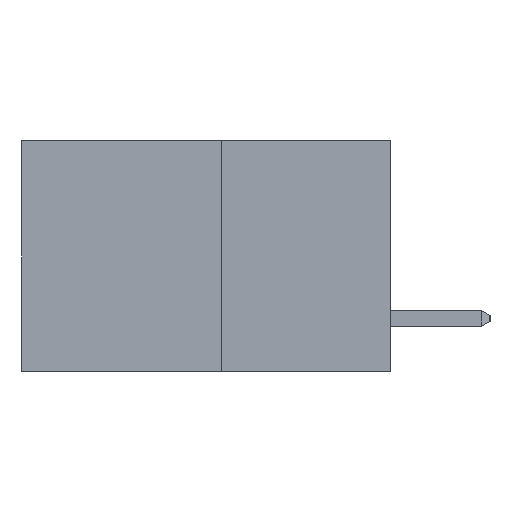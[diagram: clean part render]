
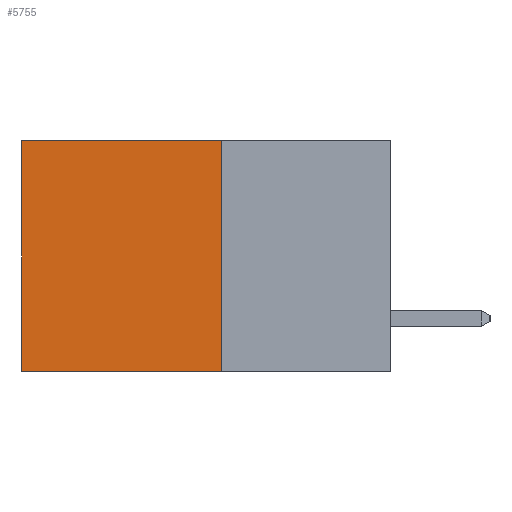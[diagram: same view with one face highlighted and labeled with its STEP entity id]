
A CAD part, left-side view. The second image highlights one B-rep face of the part: STEP entity #5755.
In plain terms, the highlighted planar face has unit normal (-1, 0, 0).
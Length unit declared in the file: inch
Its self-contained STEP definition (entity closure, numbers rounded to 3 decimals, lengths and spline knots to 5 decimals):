
#155 = DIRECTION ( 'NONE',  ( 0., 1., 0. ) ) ;
#270 = CARTESIAN_POINT ( 'NONE',  ( 0.277, 0.27, 0. ) ) ;
#315 = LINE ( 'NONE', #9768, #25990 ) ;
#1036 = VERTEX_POINT ( 'NONE', #10169 ) ;
#1504 = CARTESIAN_POINT ( 'NONE',  ( 0.277, 0.27, -0.37 ) ) ;
#3182 = ORIENTED_EDGE ( 'NONE', *, *, #17517, .T. ) ;
#3248 = EDGE_CURVE ( 'NONE', #22385, #1036, #15420, .T. ) ;
#3635 = LINE ( 'NONE', #24798, #19124 ) ;
#3652 = DIRECTION ( 'NONE',  ( 1., 0., 0. ) ) ;
#5755 = ADVANCED_FACE ( 'NONE', ( #24668 ), #13770, .F. ) ;
#6128 = ORIENTED_EDGE ( 'NONE', *, *, #3248, .T. ) ;
#7968 = DIRECTION ( 'NONE',  ( 0., 0., -1. ) ) ;
#8772 = VERTEX_POINT ( 'NONE', #22803 ) ;
#8981 = AXIS2_PLACEMENT_3D ( 'NONE', #1504, #3652, #17807 ) ;
#9768 = CARTESIAN_POINT ( 'NONE',  ( 0.277, 0.27, -0.37 ) ) ;
#10169 = CARTESIAN_POINT ( 'NONE',  ( 0.277, 0.59, 0. ) ) ;
#10907 = EDGE_CURVE ( 'NONE', #22385, #12921, #315, .T. ) ;
#12921 = VERTEX_POINT ( 'NONE', #14596 ) ;
#13770 = PLANE ( 'NONE',  #8981 ) ;
#14596 = CARTESIAN_POINT ( 'NONE',  ( 0.277, 0.27, -0.37 ) ) ;
#14891 = DIRECTION ( 'NONE',  ( 0., 1., 0. ) ) ;
#15420 = LINE ( 'NONE', #270, #25372 ) ;
#17517 = EDGE_CURVE ( 'NONE', #1036, #8772, #21435, .T. ) ;
#17807 = DIRECTION ( 'NONE',  ( 0., 0., -1. ) ) ;
#18871 = ORIENTED_EDGE ( 'NONE', *, *, #10907, .F. ) ;
#19124 = VECTOR ( 'NONE', #14891, 39.37008 ) ;
#19282 = EDGE_LOOP ( 'NONE', ( #3182, #23021, #18871, #6128 ) ) ;
#19975 = CARTESIAN_POINT ( 'NONE',  ( 0.277, 0.59, -0.37 ) ) ;
#21435 = LINE ( 'NONE', #19975, #26098 ) ;
#21573 = EDGE_CURVE ( 'NONE', #12921, #8772, #3635, .T. ) ;
#22385 = VERTEX_POINT ( 'NONE', #25541 ) ;
#22803 = CARTESIAN_POINT ( 'NONE',  ( 0.277, 0.59, -0.37 ) ) ;
#23021 = ORIENTED_EDGE ( 'NONE', *, *, #21573, .F. ) ;
#23713 = DIRECTION ( 'NONE',  ( 0., 0., -1. ) ) ;
#24668 = FACE_OUTER_BOUND ( 'NONE', #19282, .T. ) ;
#24798 = CARTESIAN_POINT ( 'NONE',  ( 0.277, 0.27, -0.37 ) ) ;
#25372 = VECTOR ( 'NONE', #155, 39.37008 ) ;
#25541 = CARTESIAN_POINT ( 'NONE',  ( 0.277, 0.27, 0. ) ) ;
#25990 = VECTOR ( 'NONE', #23713, 39.37008 ) ;
#26098 = VECTOR ( 'NONE', #7968, 39.37008 ) ;
